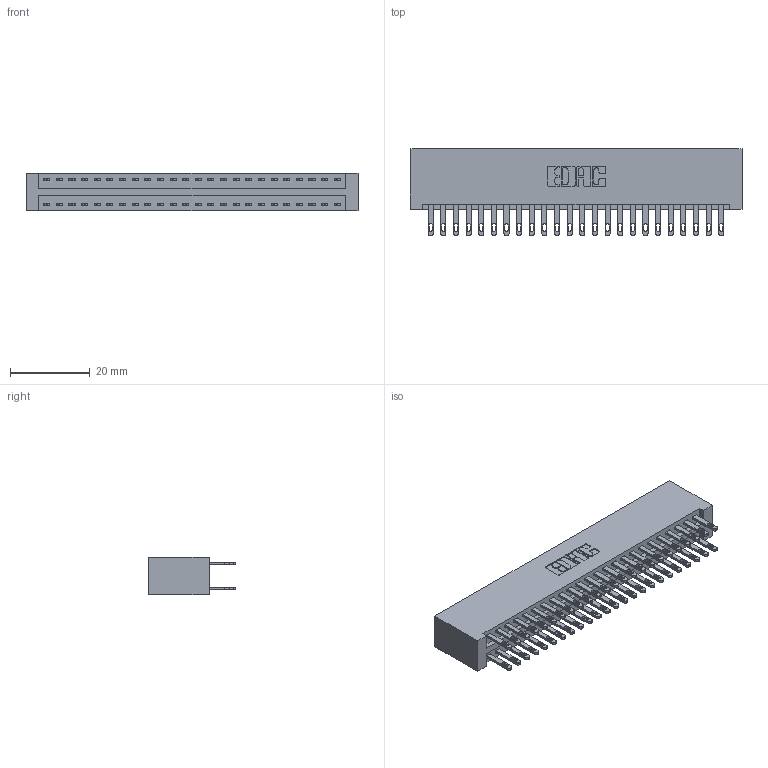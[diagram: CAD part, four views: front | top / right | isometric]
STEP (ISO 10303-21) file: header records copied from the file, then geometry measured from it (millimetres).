
FILE_DESCRIPTION (( 'STEP AP203' ), '1' );
FILE_NAME ('346-048-500-201.STEP', '2022-05-20T20:49:55', ( '' ), ( '' ), 'SwSTEP 2.0', 'SolidWorks 2020', '' );
FILE_SCHEMA (( 'CONFIG_CONTROL_DESIGN' ));
Length unit declared in the file: inch
Products named in the file (3): 346-048-500-201; 346 Part_No Mounting Lugs; 345-292-001_345-293-100
Assembly tree (49 placements, depth 2):
  346-048-500-201
    346 Part_No Mounting Lugs
    345-292-001_345-293-100  x48
Bounding box: 83.44 x 21.84 x 9.4 mm (x, y, z)
Volume: 8716.5 mm3; surface area: 12364.1 mm2
Topology: 49 solids, 49 shells, 2418 faces, 7361 edges, 4906 vertices
Faces by surface type: plane 1464, cylinder 954
Entity records: 17739 total; most frequent: CARTESIAN_POINT 2944, ORIENTED_EDGE 2878, DIRECTION 2643, EDGE_CURVE 1439, VECTOR 1215, LINE 1215, VERTEX_POINT 958, AXIS2_PLACEMENT_3D 714
